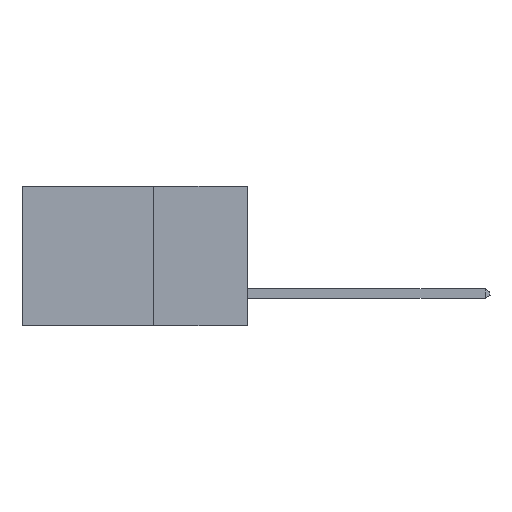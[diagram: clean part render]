
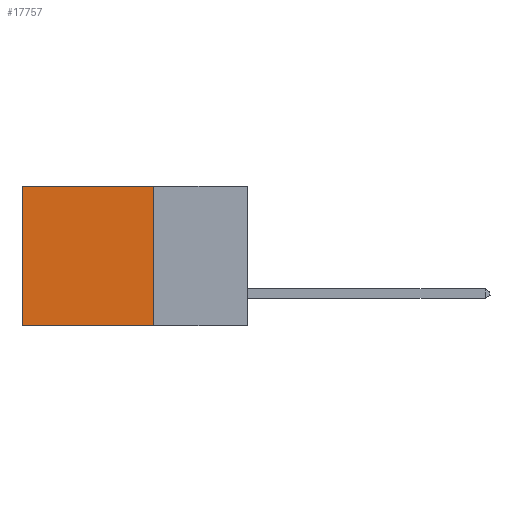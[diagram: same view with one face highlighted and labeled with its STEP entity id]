
A CAD part, left-side view. The second image highlights one B-rep face of the part: STEP entity #17757.
In plain terms, the highlighted planar face has unit normal (-1, 0, 0).
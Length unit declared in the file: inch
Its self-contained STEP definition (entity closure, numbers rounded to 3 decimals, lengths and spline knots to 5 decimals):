
#1524 = DIRECTION ( 'NONE',  ( 0., 0., -1. ) ) ;
#2836 = CARTESIAN_POINT ( 'NONE',  ( 0.298, 0.25, 0. ) ) ;
#3586 = VERTEX_POINT ( 'NONE', #16887 ) ;
#4638 = CARTESIAN_POINT ( 'NONE',  ( 0.298, 0.25, 0. ) ) ;
#4942 = CARTESIAN_POINT ( 'NONE',  ( 0.298, 0.25, -0.37 ) ) ;
#6200 = VECTOR ( 'NONE', #9756, 39.37008 ) ;
#6207 = ORIENTED_EDGE ( 'NONE', *, *, #6481, .F. ) ;
#6284 = EDGE_CURVE ( 'NONE', #6913, #7609, #13253, .T. ) ;
#6395 = CARTESIAN_POINT ( 'NONE',  ( 0.298, 0.6, -0.37 ) ) ;
#6423 = ORIENTED_EDGE ( 'NONE', *, *, #6284, .T. ) ;
#6481 = EDGE_CURVE ( 'NONE', #3586, #8461, #18274, .T. ) ;
#6653 = CARTESIAN_POINT ( 'NONE',  ( 0.298, 0.25, -0.37 ) ) ;
#6913 = VERTEX_POINT ( 'NONE', #16875 ) ;
#6943 = EDGE_CURVE ( 'NONE', #8461, #7609, #16089, .T. ) ;
#7238 = CARTESIAN_POINT ( 'NONE',  ( 0.298, 0.25, 0. ) ) ;
#7457 = VECTOR ( 'NONE', #12298, 39.37008 ) ;
#7609 = VERTEX_POINT ( 'NONE', #6395 ) ;
#8461 = VERTEX_POINT ( 'NONE', #6653 ) ;
#8685 = CARTESIAN_POINT ( 'NONE',  ( 0.298, 0.6, 0. ) ) ;
#8747 = VECTOR ( 'NONE', #1524, 39.37008 ) ;
#9756 = DIRECTION ( 'NONE',  ( 0., 0., -1. ) ) ;
#12275 = LINE ( 'NONE', #7238, #7457 ) ;
#12298 = DIRECTION ( 'NONE',  ( 0., 1., 0. ) ) ;
#12731 = ORIENTED_EDGE ( 'NONE', *, *, #6943, .F. ) ;
#13253 = LINE ( 'NONE', #8685, #8747 ) ;
#13487 = DIRECTION ( 'NONE',  ( 0., 0., -1. ) ) ;
#13636 = PLANE ( 'NONE',  #19493 ) ;
#16089 = LINE ( 'NONE', #4942, #19714 ) ;
#16875 = CARTESIAN_POINT ( 'NONE',  ( 0.298, 0.6, 0. ) ) ;
#16887 = CARTESIAN_POINT ( 'NONE',  ( 0.298, 0.25, 0. ) ) ;
#17594 = DIRECTION ( 'NONE',  ( 0., 1., 0. ) ) ;
#17757 = ADVANCED_FACE ( 'NONE', ( #19731 ), #13636, .F. ) ;
#18274 = LINE ( 'NONE', #4638, #6200 ) ;
#19493 = AXIS2_PLACEMENT_3D ( 'NONE', #2836, #20858, #13487 ) ;
#19714 = VECTOR ( 'NONE', #17594, 39.37008 ) ;
#19731 = FACE_OUTER_BOUND ( 'NONE', #22730, .T. ) ;
#19850 = ORIENTED_EDGE ( 'NONE', *, *, #21199, .T. ) ;
#20858 = DIRECTION ( 'NONE',  ( 1., 0., 0. ) ) ;
#21199 = EDGE_CURVE ( 'NONE', #3586, #6913, #12275, .T. ) ;
#22730 = EDGE_LOOP ( 'NONE', ( #6423, #12731, #6207, #19850 ) ) ;
